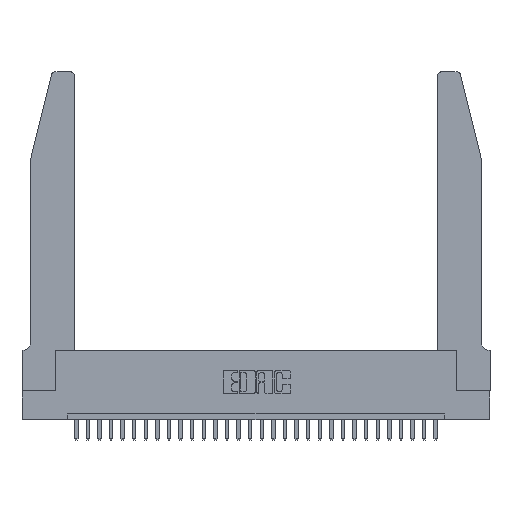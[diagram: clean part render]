
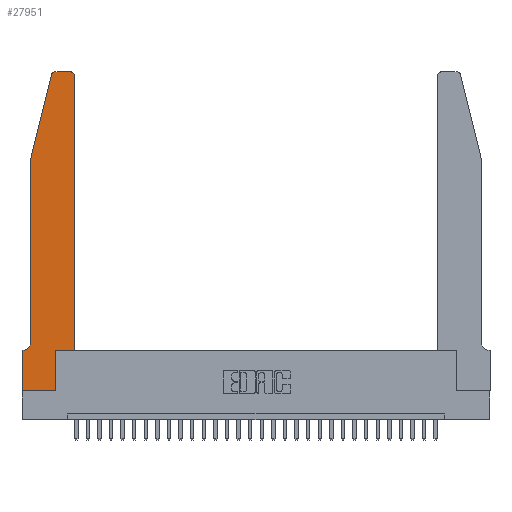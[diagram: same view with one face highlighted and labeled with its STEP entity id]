
A CAD part, top view. The second image highlights one B-rep face of the part: STEP entity #27951.
In plain terms, the highlighted planar face has unit normal (0, 0, 1).
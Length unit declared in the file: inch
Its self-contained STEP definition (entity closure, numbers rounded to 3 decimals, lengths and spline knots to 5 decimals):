
#255 = DIRECTION ( 'NONE',  ( -1., 0., 0. ) ) ;
#320 = LINE ( 'NONE', #27186, #13521 ) ;
#568 = CARTESIAN_POINT ( 'NONE',  ( 0.2865, 0.35, 0.37 ) ) ;
#607 = EDGE_CURVE ( 'NONE', #1665, #11339, #28576, .T. ) ;
#732 = VERTEX_POINT ( 'NONE', #23578 ) ;
#911 = LINE ( 'NONE', #23339, #25038 ) ;
#1081 = ORIENTED_EDGE ( 'NONE', *, *, #8151, .T. ) ;
#1364 = VECTOR ( 'NONE', #6248, 39.37008 ) ;
#1391 = VECTOR ( 'NONE', #6860, 39.37008 ) ;
#1665 = VERTEX_POINT ( 'NONE', #568 ) ;
#1691 = DIRECTION ( 'NONE',  ( 1., 0., 0. ) ) ;
#1793 = CARTESIAN_POINT ( 'NONE',  ( 0.4505, 0.35, 0.37 ) ) ;
#1871 = VERTEX_POINT ( 'NONE', #20493 ) ;
#1898 = CARTESIAN_POINT ( 'NONE',  ( 0.0755, 2., 0.37 ) ) ;
#2142 = CARTESIAN_POINT ( 'NONE',  ( 0.2865, 0.35, 0.37 ) ) ;
#2181 = ORIENTED_EDGE ( 'NONE', *, *, #26401, .T. ) ;
#2982 = CARTESIAN_POINT ( 'NONE',  ( 0.4505, 2.72, 0.37 ) ) ;
#3000 = AXIS2_PLACEMENT_3D ( 'NONE', #17206, #17300, #21794 ) ;
#3541 = ORIENTED_EDGE ( 'NONE', *, *, #18789, .T. ) ;
#4862 = ORIENTED_EDGE ( 'NONE', *, *, #8499, .T. ) ;
#5622 = CARTESIAN_POINT ( 'NONE',  ( 0.0055, 0.35, 0.37 ) ) ;
#6248 = DIRECTION ( 'NONE',  ( 0., -1., 0. ) ) ;
#6327 = CARTESIAN_POINT ( 'NONE',  ( 0., 0., 0.37 ) ) ;
#6406 = LINE ( 'NONE', #6327, #15565 ) ;
#6860 = DIRECTION ( 'NONE',  ( 0., 1., 0. ) ) ;
#7179 = AXIS2_PLACEMENT_3D ( 'NONE', #18870, #21197, #11906 ) ;
#7872 = LINE ( 'NONE', #1793, #11507 ) ;
#8029 = CARTESIAN_POINT ( 'NONE',  ( 0.4505, 0.35, 0.37 ) ) ;
#8151 = EDGE_CURVE ( 'NONE', #27204, #28387, #27954, .T. ) ;
#8401 = VERTEX_POINT ( 'NONE', #2982 ) ;
#8499 = EDGE_CURVE ( 'NONE', #11339, #8401, #7872, .T. ) ;
#8501 = EDGE_CURVE ( 'NONE', #28387, #1871, #29788, .T. ) ;
#8697 = CARTESIAN_POINT ( 'NONE',  ( 0., 0., 0.37 ) ) ;
#9549 = ORIENTED_EDGE ( 'NONE', *, *, #607, .T. ) ;
#9716 = EDGE_CURVE ( 'NONE', #1871, #24187, #15875, .T. ) ;
#9972 = PLANE ( 'NONE',  #3000 ) ;
#10382 = ORIENTED_EDGE ( 'NONE', *, *, #8501, .T. ) ;
#10787 = ORIENTED_EDGE ( 'NONE', *, *, #20742, .T. ) ;
#10917 = VERTEX_POINT ( 'NONE', #12328 ) ;
#11008 = DIRECTION ( 'NONE',  ( 0., 1., 0. ) ) ;
#11339 = VERTEX_POINT ( 'NONE', #8029 ) ;
#11477 = VERTEX_POINT ( 'NONE', #18394 ) ;
#11507 = VECTOR ( 'NONE', #11008, 39.37008 ) ;
#11906 = DIRECTION ( 'NONE',  ( 1., 0., 0. ) ) ;
#12328 = CARTESIAN_POINT ( 'NONE',  ( 0.284, 2.75, 0.37 ) ) ;
#12403 = VERTEX_POINT ( 'NONE', #18521 ) ;
#13399 = DIRECTION ( 'NONE',  ( 0., 0., 1. ) ) ;
#13426 = EDGE_CURVE ( 'NONE', #8401, #732, #17078, .T. ) ;
#13521 = VECTOR ( 'NONE', #15379, 39.37008 ) ;
#13847 = FACE_OUTER_BOUND ( 'NONE', #22254, .T. ) ;
#14122 = DIRECTION ( 'NONE',  ( 1., 0., 0. ) ) ;
#14656 = CARTESIAN_POINT ( 'NONE',  ( 0.0755, 2., 0.37 ) ) ;
#15096 = VECTOR ( 'NONE', #14122, 39.37008 ) ;
#15379 = DIRECTION ( 'NONE',  ( -1., 0., 0. ) ) ;
#15565 = VECTOR ( 'NONE', #1691, 39.37008 ) ;
#15875 = CIRCLE ( 'NONE', #28215, 0.07 ) ;
#16016 = ORIENTED_EDGE ( 'NONE', *, *, #24489, .T. ) ;
#16174 = CARTESIAN_POINT ( 'NONE',  ( 0.4505, 0.35, 0.37 ) ) ;
#17078 = CIRCLE ( 'NONE', #27080, 0.03 ) ;
#17206 = CARTESIAN_POINT ( 'NONE',  ( 0., 0.35, 0.37 ) ) ;
#17300 = DIRECTION ( 'NONE',  ( 0., 0., 1. ) ) ;
#17724 = ORIENTED_EDGE ( 'NONE', *, *, #9716, .T. ) ;
#17828 = LINE ( 'NONE', #8697, #1364 ) ;
#18046 = DIRECTION ( 'NONE',  ( 0., -1., 0. ) ) ;
#18394 = CARTESIAN_POINT ( 'NONE',  ( 0.2865, 0., 0.37 ) ) ;
#18521 = CARTESIAN_POINT ( 'NONE',  ( 0., 0., 0.37 ) ) ;
#18789 = EDGE_CURVE ( 'NONE', #19916, #12403, #17828, .T. ) ;
#18870 = CARTESIAN_POINT ( 'NONE',  ( 0.284, 2.72, 0.37 ) ) ;
#18920 = CARTESIAN_POINT ( 'NONE',  ( 0.25487, 2.72718, 0.37 ) ) ;
#19916 = VERTEX_POINT ( 'NONE', #20039 ) ;
#20039 = CARTESIAN_POINT ( 'NONE',  ( 0., 0.35, 0.37 ) ) ;
#20120 = ORIENTED_EDGE ( 'NONE', *, *, #13426, .T. ) ;
#20493 = CARTESIAN_POINT ( 'NONE',  ( 0.0755, 0.42, 0.37 ) ) ;
#20742 = EDGE_CURVE ( 'NONE', #10917, #27204, #21992, .T. ) ;
#21197 = DIRECTION ( 'NONE',  ( 0., 0., 1. ) ) ;
#21374 = DIRECTION ( 'NONE',  ( -1., 0., 0. ) ) ;
#21794 = DIRECTION ( 'NONE',  ( 1., 0., 0. ) ) ;
#21992 = CIRCLE ( 'NONE', #7179, 0.03 ) ;
#22254 = EDGE_LOOP ( 'NONE', ( #2181, #10787, #1081, #10382, #17724, #16016, #3541, #27045, #28831, #9549, #4862, #20120 ) ) ;
#22311 = EDGE_CURVE ( 'NONE', #11477, #1665, #28466, .T. ) ;
#22368 = CARTESIAN_POINT ( 'NONE',  ( 0.0755, 2., 0.37 ) ) ;
#22860 = DIRECTION ( 'NONE',  ( 1., 0., 0. ) ) ;
#23187 = CARTESIAN_POINT ( 'NONE',  ( 0.0055, 0.42, 0.37 ) ) ;
#23339 = CARTESIAN_POINT ( 'NONE',  ( 0.0755, 0.35, 0.37 ) ) ;
#23566 = VECTOR ( 'NONE', #24715, 39.37008 ) ;
#23578 = CARTESIAN_POINT ( 'NONE',  ( 0.4205, 2.75, 0.37 ) ) ;
#24187 = VERTEX_POINT ( 'NONE', #5622 ) ;
#24310 = EDGE_CURVE ( 'NONE', #12403, #11477, #6406, .T. ) ;
#24489 = EDGE_CURVE ( 'NONE', #24187, #19916, #911, .T. ) ;
#24715 = DIRECTION ( 'NONE',  ( -0.239, -0.971, 0. ) ) ;
#25038 = VECTOR ( 'NONE', #255, 39.37008 ) ;
#26031 = DIRECTION ( 'NONE',  ( 0., 0., -1. ) ) ;
#26401 = EDGE_CURVE ( 'NONE', #732, #10917, #320, .T. ) ;
#27045 = ORIENTED_EDGE ( 'NONE', *, *, #24310, .T. ) ;
#27080 = AXIS2_PLACEMENT_3D ( 'NONE', #27329, #13399, #22860 ) ;
#27186 = CARTESIAN_POINT ( 'NONE',  ( 0.2605, 2.75, 0.37 ) ) ;
#27204 = VERTEX_POINT ( 'NONE', #18920 ) ;
#27329 = CARTESIAN_POINT ( 'NONE',  ( 0.4205, 2.72, 0.37 ) ) ;
#27951 = ADVANCED_FACE ( 'NONE', ( #13847 ), #9972, .T. ) ;
#27954 = LINE ( 'NONE', #22368, #23566 ) ;
#28215 = AXIS2_PLACEMENT_3D ( 'NONE', #23187, #26031, #21374 ) ;
#28387 = VERTEX_POINT ( 'NONE', #14656 ) ;
#28466 = LINE ( 'NONE', #2142, #1391 ) ;
#28576 = LINE ( 'NONE', #16174, #15096 ) ;
#28677 = VECTOR ( 'NONE', #18046, 39.37008 ) ;
#28831 = ORIENTED_EDGE ( 'NONE', *, *, #22311, .T. ) ;
#29788 = LINE ( 'NONE', #1898, #28677 ) ;
